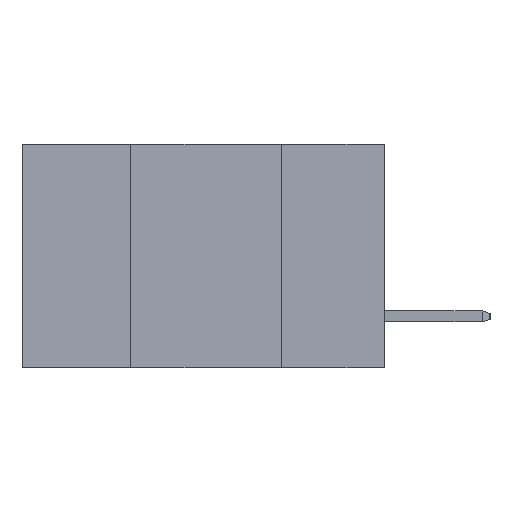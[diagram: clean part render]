
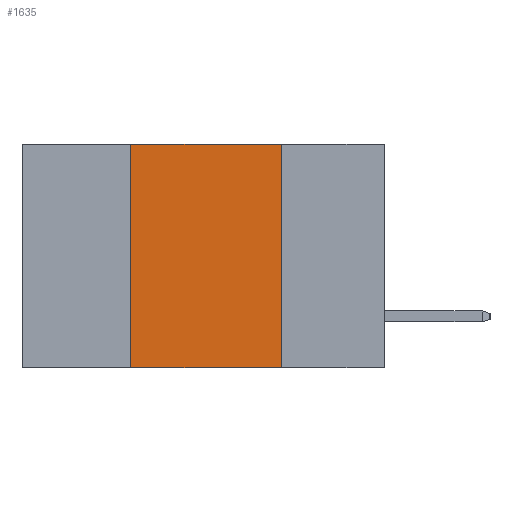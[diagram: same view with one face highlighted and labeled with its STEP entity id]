
A CAD part, left-side view. The second image highlights one B-rep face of the part: STEP entity #1635.
In plain terms, the highlighted planar face has unit normal (-1, 0, 0).
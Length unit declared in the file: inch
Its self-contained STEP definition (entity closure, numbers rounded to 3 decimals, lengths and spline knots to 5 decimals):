
#139 = CARTESIAN_POINT ( 'NONE',  ( 0., 0.42, 0. ) ) ;
#372 = ORIENTED_EDGE ( 'NONE', *, *, #14487, .T. ) ;
#495 = VECTOR ( 'NONE', #14505, 39.37008 ) ;
#538 = EDGE_CURVE ( 'NONE', #7893, #13864, #7423, .T. ) ;
#1303 = LINE ( 'NONE', #9947, #495 ) ;
#1635 = ADVANCED_FACE ( 'NONE', ( #3828 ), #15141, .F. ) ;
#2052 = DIRECTION ( 'NONE',  ( 0., 0., 1. ) ) ;
#2254 = EDGE_CURVE ( 'NONE', #13116, #11173, #5503, .T. ) ;
#3371 = ORIENTED_EDGE ( 'NONE', *, *, #538, .F. ) ;
#3421 = CARTESIAN_POINT ( 'NONE',  ( 0., 0.6, 0. ) ) ;
#3828 = FACE_OUTER_BOUND ( 'NONE', #7332, .T. ) ;
#4049 = VECTOR ( 'NONE', #8558, 39.37008 ) ;
#5277 = DIRECTION ( 'NONE',  ( 1., 0., 0. ) ) ;
#5503 = LINE ( 'NONE', #10661, #8002 ) ;
#6590 = ORIENTED_EDGE ( 'NONE', *, *, #12226, .F. ) ;
#7332 = EDGE_LOOP ( 'NONE', ( #10203, #6590, #3371, #372 ) ) ;
#7423 = LINE ( 'NONE', #9415, #11349 ) ;
#7893 = VERTEX_POINT ( 'NONE', #10331 ) ;
#7933 = CARTESIAN_POINT ( 'NONE',  ( 0., 0.17, 0. ) ) ;
#8002 = VECTOR ( 'NONE', #14933, 39.37008 ) ;
#8558 = DIRECTION ( 'NONE',  ( 0., -1., 0. ) ) ;
#9415 = CARTESIAN_POINT ( 'NONE',  ( 0., 0.42, 0. ) ) ;
#9700 = CARTESIAN_POINT ( 'NONE',  ( 0., 0.6, 0. ) ) ;
#9757 = AXIS2_PLACEMENT_3D ( 'NONE', #3421, #5277, #13571 ) ;
#9947 = CARTESIAN_POINT ( 'NONE',  ( 0., 0.6, -0.37 ) ) ;
#10203 = ORIENTED_EDGE ( 'NONE', *, *, #2254, .F. ) ;
#10331 = CARTESIAN_POINT ( 'NONE',  ( 0., 0.42, -0.37 ) ) ;
#10661 = CARTESIAN_POINT ( 'NONE',  ( 0., 0.17, 0. ) ) ;
#11015 = CARTESIAN_POINT ( 'NONE',  ( 0., 0.17, -0.37 ) ) ;
#11173 = VERTEX_POINT ( 'NONE', #11015 ) ;
#11349 = VECTOR ( 'NONE', #2052, 39.37008 ) ;
#12226 = EDGE_CURVE ( 'NONE', #13864, #13116, #13488, .T. ) ;
#13116 = VERTEX_POINT ( 'NONE', #7933 ) ;
#13488 = LINE ( 'NONE', #9700, #4049 ) ;
#13571 = DIRECTION ( 'NONE',  ( 0., 0., -1. ) ) ;
#13864 = VERTEX_POINT ( 'NONE', #139 ) ;
#14487 = EDGE_CURVE ( 'NONE', #7893, #11173, #1303, .T. ) ;
#14505 = DIRECTION ( 'NONE',  ( 0., -1., 0. ) ) ;
#14933 = DIRECTION ( 'NONE',  ( 0., 0., -1. ) ) ;
#15141 = PLANE ( 'NONE',  #9757 ) ;
